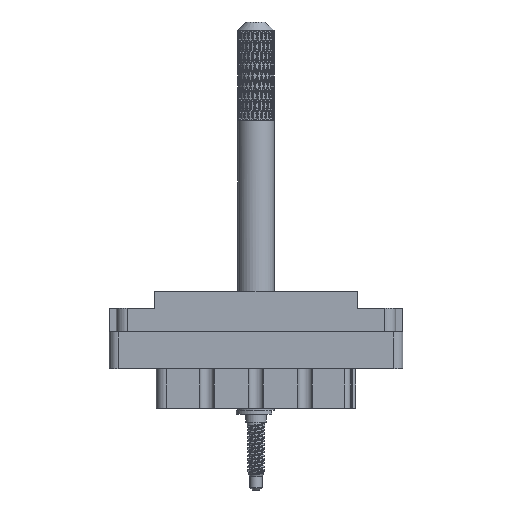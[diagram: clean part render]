
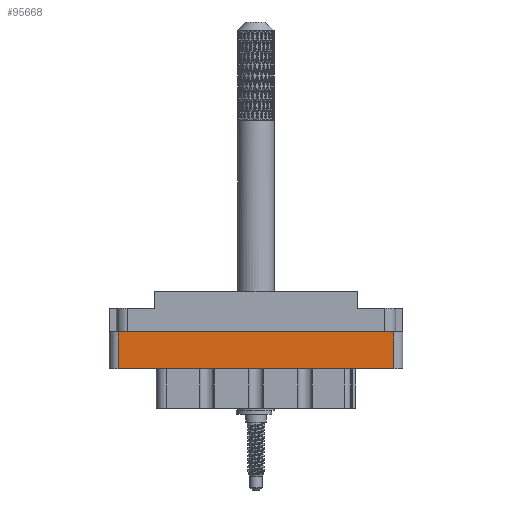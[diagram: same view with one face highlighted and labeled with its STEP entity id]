
A CAD part, front view. The second image highlights one B-rep face of the part: STEP entity #95668.
In plain terms, the highlighted planar face has unit normal (0, -1, 0).
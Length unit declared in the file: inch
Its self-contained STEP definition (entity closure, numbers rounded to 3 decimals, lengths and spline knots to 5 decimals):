
#3431 = VECTOR ( 'NONE', #12723, 39.37008 ) ;
#4795 = VERTEX_POINT ( 'NONE', #11118 ) ;
#7737 = VERTEX_POINT ( 'NONE', #82924 ) ;
#11118 = CARTESIAN_POINT ( 'NONE',  ( 0.938, -0.438, -0.529 ) ) ;
#12723 = DIRECTION ( 'NONE',  ( 0., 0., 1. ) ) ;
#19462 = CARTESIAN_POINT ( 'NONE',  ( 0., -0.438, -0.529 ) ) ;
#22431 = LINE ( 'NONE', #19462, #52808 ) ;
#33807 = DIRECTION ( 'NONE',  ( 0., -1., 0. ) ) ;
#34460 = DIRECTION ( 'NONE',  ( 0., 0., -1. ) ) ;
#34512 = ORIENTED_EDGE ( 'NONE', *, *, #61290, .T. ) ;
#36517 = VERTEX_POINT ( 'NONE', #43147 ) ;
#38105 = EDGE_CURVE ( 'NONE', #4795, #7737, #22431, .T. ) ;
#39798 = CARTESIAN_POINT ( 'NONE',  ( -0.938, -0.438, -0.798 ) ) ;
#42509 = EDGE_LOOP ( 'NONE', ( #61078, #53722, #76809, #34512 ) ) ;
#43147 = CARTESIAN_POINT ( 'NONE',  ( -0.938, -0.438, -0.277 ) ) ;
#44637 = DIRECTION ( 'NONE',  ( 1., 0., 0. ) ) ;
#46408 = EDGE_CURVE ( 'NONE', #36517, #99940, #50756, .T. ) ;
#50668 = DIRECTION ( 'NONE',  ( -1., 0., 0. ) ) ;
#50756 = LINE ( 'NONE', #83007, #51917 ) ;
#51917 = VECTOR ( 'NONE', #44637, 39.37008 ) ;
#52808 = VECTOR ( 'NONE', #50668, 39.37008 ) ;
#53722 = ORIENTED_EDGE ( 'NONE', *, *, #86747, .T. ) ;
#57233 = PLANE ( 'NONE',  #96506 ) ;
#57466 = LINE ( 'NONE', #39798, #91467 ) ;
#61078 = ORIENTED_EDGE ( 'NONE', *, *, #46408, .F. ) ;
#61290 = EDGE_CURVE ( 'NONE', #4795, #99940, #61706, .T. ) ;
#61706 = LINE ( 'NONE', #98569, #3431 ) ;
#63929 = DIRECTION ( 'NONE',  ( 0., 0., -1. ) ) ;
#73219 = CARTESIAN_POINT ( 'NONE',  ( -1., -0.438, -0.798 ) ) ;
#76809 = ORIENTED_EDGE ( 'NONE', *, *, #38105, .F. ) ;
#79652 = FACE_OUTER_BOUND ( 'NONE', #42509, .T. ) ;
#82924 = CARTESIAN_POINT ( 'NONE',  ( -0.938, -0.438, -0.529 ) ) ;
#83007 = CARTESIAN_POINT ( 'NONE',  ( 0., -0.438, -0.277 ) ) ;
#86747 = EDGE_CURVE ( 'NONE', #36517, #7737, #57466, .T. ) ;
#91467 = VECTOR ( 'NONE', #63929, 39.37008 ) ;
#94625 = CARTESIAN_POINT ( 'NONE',  ( 0.938, -0.438, -0.277 ) ) ;
#95668 = ADVANCED_FACE ( 'NONE', ( #79652 ), #57233, .T. ) ;
#96506 = AXIS2_PLACEMENT_3D ( 'NONE', #73219, #33807, #34460 ) ;
#98569 = CARTESIAN_POINT ( 'NONE',  ( 0.938, -0.438, -0.798 ) ) ;
#99940 = VERTEX_POINT ( 'NONE', #94625 ) ;
